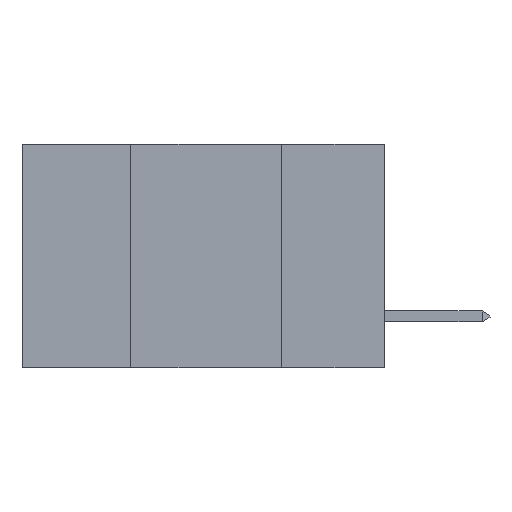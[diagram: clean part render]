
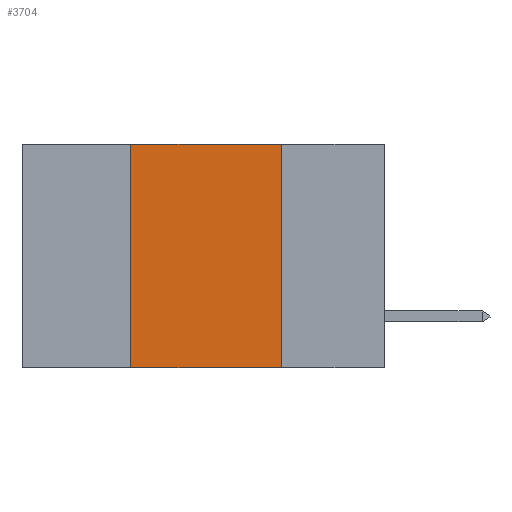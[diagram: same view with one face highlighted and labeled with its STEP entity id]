
A CAD part, left-side view. The second image highlights one B-rep face of the part: STEP entity #3704.
In plain terms, the highlighted planar face has unit normal (-1, 0, 0).
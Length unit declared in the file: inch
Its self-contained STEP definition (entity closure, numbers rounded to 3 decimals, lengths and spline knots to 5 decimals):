
#80 = ORIENTED_EDGE ( 'NONE', *, *, #7351, .F. ) ;
#258 = VECTOR ( 'NONE', #2716, 39.37008 ) ;
#482 = CARTESIAN_POINT ( 'NONE',  ( 0., 0.6, 0. ) ) ;
#723 = CARTESIAN_POINT ( 'NONE',  ( 0., 0.42, -0.37 ) ) ;
#1231 = CARTESIAN_POINT ( 'NONE',  ( 0., 0.42, 0. ) ) ;
#1275 = CARTESIAN_POINT ( 'NONE',  ( 0., 0.17, 0. ) ) ;
#2115 = EDGE_CURVE ( 'NONE', #9170, #5113, #12545, .T. ) ;
#2177 = ORIENTED_EDGE ( 'NONE', *, *, #2115, .T. ) ;
#2716 = DIRECTION ( 'NONE',  ( 0., 0., 1. ) ) ;
#3044 = VECTOR ( 'NONE', #5112, 39.37008 ) ;
#3451 = CARTESIAN_POINT ( 'NONE',  ( 0., 0.17, 0. ) ) ;
#3704 = ADVANCED_FACE ( 'NONE', ( #12467 ), #14550, .F. ) ;
#5034 = DIRECTION ( 'NONE',  ( 1., 0., 0. ) ) ;
#5112 = DIRECTION ( 'NONE',  ( 0., 0., -1. ) ) ;
#5113 = VERTEX_POINT ( 'NONE', #9325 ) ;
#5403 = VECTOR ( 'NONE', #19158, 39.37008 ) ;
#5568 = AXIS2_PLACEMENT_3D ( 'NONE', #482, #5034, #12951 ) ;
#7351 = EDGE_CURVE ( 'NONE', #8637, #5113, #11577, .T. ) ;
#7820 = LINE ( 'NONE', #1231, #258 ) ;
#8101 = DIRECTION ( 'NONE',  ( 0., -1., 0. ) ) ;
#8445 = VECTOR ( 'NONE', #8101, 39.37008 ) ;
#8637 = VERTEX_POINT ( 'NONE', #1275 ) ;
#8949 = CARTESIAN_POINT ( 'NONE',  ( 0., 0.42, 0. ) ) ;
#8964 = EDGE_LOOP ( 'NONE', ( #80, #10715, #17346, #2177 ) ) ;
#9170 = VERTEX_POINT ( 'NONE', #723 ) ;
#9325 = CARTESIAN_POINT ( 'NONE',  ( 0., 0.17, -0.37 ) ) ;
#9520 = LINE ( 'NONE', #17534, #5403 ) ;
#10304 = EDGE_CURVE ( 'NONE', #9170, #11006, #7820, .T. ) ;
#10621 = EDGE_CURVE ( 'NONE', #11006, #8637, #9520, .T. ) ;
#10715 = ORIENTED_EDGE ( 'NONE', *, *, #10621, .F. ) ;
#11006 = VERTEX_POINT ( 'NONE', #8949 ) ;
#11284 = CARTESIAN_POINT ( 'NONE',  ( 0., 0.6, -0.37 ) ) ;
#11577 = LINE ( 'NONE', #3451, #3044 ) ;
#12467 = FACE_OUTER_BOUND ( 'NONE', #8964, .T. ) ;
#12545 = LINE ( 'NONE', #11284, #8445 ) ;
#12951 = DIRECTION ( 'NONE',  ( 0., 0., -1. ) ) ;
#14550 = PLANE ( 'NONE',  #5568 ) ;
#17346 = ORIENTED_EDGE ( 'NONE', *, *, #10304, .F. ) ;
#17534 = CARTESIAN_POINT ( 'NONE',  ( 0., 0.6, 0. ) ) ;
#19158 = DIRECTION ( 'NONE',  ( 0., -1., 0. ) ) ;
